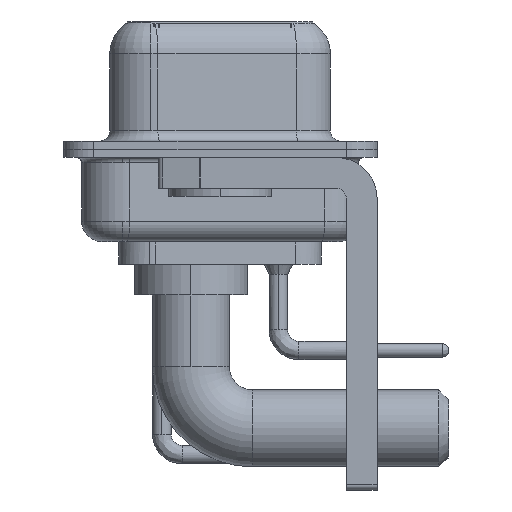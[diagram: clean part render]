
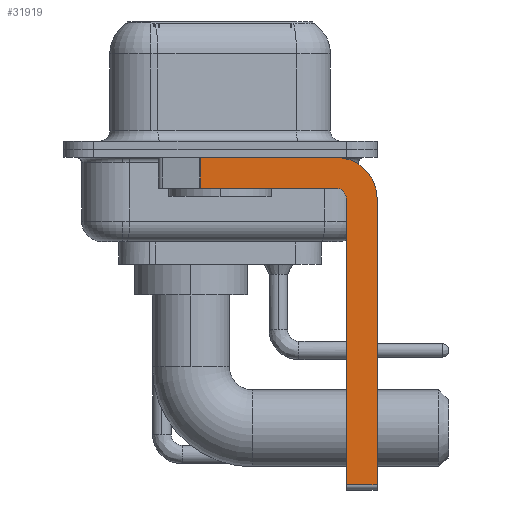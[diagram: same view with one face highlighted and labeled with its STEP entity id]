
A CAD part, left-side view. The second image highlights one B-rep face of the part: STEP entity #31919.
In plain terms, the highlighted planar face has unit normal (-1, 0, 0).
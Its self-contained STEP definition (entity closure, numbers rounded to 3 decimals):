
#536 = ORIENTED_EDGE ( 'NONE', *, *, #1992, .F. ) ;
#644 = LINE ( 'NONE', #22114, #31836 ) ;
#705 = EDGE_CURVE ( 'NONE', #6477, #29469, #1642, .T. ) ;
#1451 = LINE ( 'NONE', #20633, #13278 ) ;
#1642 = LINE ( 'NONE', #33976, #16669 ) ;
#1992 = EDGE_CURVE ( 'NONE', #21678, #9304, #644, .T. ) ;
#2795 = VERTEX_POINT ( 'NONE', #30049 ) ;
#3619 = DIRECTION ( 'NONE',  ( 0., -1., 0. ) ) ;
#3914 = DIRECTION ( 'NONE',  ( 0., 0., -1. ) ) ;
#4017 = CARTESIAN_POINT ( 'NONE',  ( -2.9, 0.978, -1.9 ) ) ;
#4258 = DIRECTION ( 'NONE',  ( 0., -1., 0. ) ) ;
#5070 = CARTESIAN_POINT ( 'NONE',  ( -2.9, -5.65, -0.4 ) ) ;
#5657 = CARTESIAN_POINT ( 'NONE',  ( -2.9, -5.65, -2.4 ) ) ;
#6477 = VERTEX_POINT ( 'NONE', #13633 ) ;
#6807 = VECTOR ( 'NONE', #4258, 1000. ) ;
#6917 = ORIENTED_EDGE ( 'NONE', *, *, #18650, .T. ) ;
#7188 = VERTEX_POINT ( 'NONE', #12040 ) ;
#7323 = VERTEX_POINT ( 'NONE', #29606 ) ;
#7463 = ORIENTED_EDGE ( 'NONE', *, *, #10530, .F. ) ;
#7941 = EDGE_CURVE ( 'NONE', #21678, #29469, #28128, .T. ) ;
#8654 = DIRECTION ( 'NONE',  ( 1., 0., 0. ) ) ;
#8659 = DIRECTION ( 'NONE',  ( 0., 0., -1. ) ) ;
#9304 = VERTEX_POINT ( 'NONE', #5070 ) ;
#9388 = CARTESIAN_POINT ( 'NONE',  ( -2.9, -5.65, -2.4 ) ) ;
#10530 = EDGE_CURVE ( 'NONE', #7188, #2795, #1451, .T. ) ;
#11984 = VECTOR ( 'NONE', #33012, 1000. ) ;
#12040 = CARTESIAN_POINT ( 'NONE',  ( -2.9, -6.15, -16.35 ) ) ;
#12248 = ORIENTED_EDGE ( 'NONE', *, *, #705, .F. ) ;
#12973 = VERTEX_POINT ( 'NONE', #30409 ) ;
#13278 = VECTOR ( 'NONE', #28708, 1000. ) ;
#13633 = CARTESIAN_POINT ( 'NONE',  ( -2.9, -5.65, -1.9 ) ) ;
#15505 = CIRCLE ( 'NONE', #32892, 0.5 ) ;
#16587 = FACE_OUTER_BOUND ( 'NONE', #25279, .T. ) ;
#16669 = VECTOR ( 'NONE', #33801, 1000. ) ;
#17984 = LINE ( 'NONE', #28363, #6807 ) ;
#18650 = EDGE_CURVE ( 'NONE', #7188, #12973, #17984, .T. ) ;
#19761 = CARTESIAN_POINT ( 'NONE',  ( -2.9, -7.65, -2.4 ) ) ;
#20441 = AXIS2_PLACEMENT_3D ( 'NONE', #5657, #27126, #30084 ) ;
#20633 = CARTESIAN_POINT ( 'NONE',  ( -2.9, -6.15, -16.6 ) ) ;
#21678 = VERTEX_POINT ( 'NONE', #25053 ) ;
#22050 = LINE ( 'NONE', #19761, #22969 ) ;
#22082 = EDGE_CURVE ( 'NONE', #9304, #7323, #28860, .T. ) ;
#22114 = CARTESIAN_POINT ( 'NONE',  ( -2.9, 3., -0.4 ) ) ;
#22599 = ORIENTED_EDGE ( 'NONE', *, *, #22082, .F. ) ;
#22969 = VECTOR ( 'NONE', #8659, 1000. ) ;
#23891 = CARTESIAN_POINT ( 'NONE',  ( -2.9, 0.978, -1.9 ) ) ;
#24048 = AXIS2_PLACEMENT_3D ( 'NONE', #32727, #8654, #3914 ) ;
#25053 = CARTESIAN_POINT ( 'NONE',  ( -2.9, 0.978, -0.4 ) ) ;
#25279 = EDGE_LOOP ( 'NONE', ( #536, #29560, #12248, #32751, #7463, #6917, #32635, #22599 ) ) ;
#25410 = DIRECTION ( 'NONE',  ( -1., 0., 0. ) ) ;
#27126 = DIRECTION ( 'NONE',  ( 1., 0., 0. ) ) ;
#27674 = EDGE_CURVE ( 'NONE', #7323, #12973, #22050, .T. ) ;
#28020 = PLANE ( 'NONE',  #24048 ) ;
#28128 = LINE ( 'NONE', #4017, #11984 ) ;
#28363 = CARTESIAN_POINT ( 'NONE',  ( -2.9, -5.65, -16.35 ) ) ;
#28708 = DIRECTION ( 'NONE',  ( 0., 0., 1. ) ) ;
#28860 = CIRCLE ( 'NONE', #20441, 2. ) ;
#29469 = VERTEX_POINT ( 'NONE', #23891 ) ;
#29560 = ORIENTED_EDGE ( 'NONE', *, *, #7941, .T. ) ;
#29606 = CARTESIAN_POINT ( 'NONE',  ( -2.9, -7.65, -2.4 ) ) ;
#30049 = CARTESIAN_POINT ( 'NONE',  ( -2.9, -6.15, -2.4 ) ) ;
#30084 = DIRECTION ( 'NONE',  ( 0., 0., -1. ) ) ;
#30347 = EDGE_CURVE ( 'NONE', #2795, #6477, #15505, .T. ) ;
#30409 = CARTESIAN_POINT ( 'NONE',  ( -2.9, -7.65, -16.35 ) ) ;
#31836 = VECTOR ( 'NONE', #3619, 1000. ) ;
#31919 = ADVANCED_FACE ( 'NONE', ( #16587 ), #28020, .F. ) ;
#32635 = ORIENTED_EDGE ( 'NONE', *, *, #27674, .F. ) ;
#32727 = CARTESIAN_POINT ( 'NONE',  ( -2.9, -5.65, -2.4 ) ) ;
#32751 = ORIENTED_EDGE ( 'NONE', *, *, #30347, .F. ) ;
#32892 = AXIS2_PLACEMENT_3D ( 'NONE', #9388, #25410, #33454 ) ;
#33012 = DIRECTION ( 'NONE',  ( 0., 0., -1. ) ) ;
#33454 = DIRECTION ( 'NONE',  ( 0., 0., 1. ) ) ;
#33801 = DIRECTION ( 'NONE',  ( 0., 1., 0. ) ) ;
#33976 = CARTESIAN_POINT ( 'NONE',  ( -2.9, -5.65, -1.9 ) ) ;
